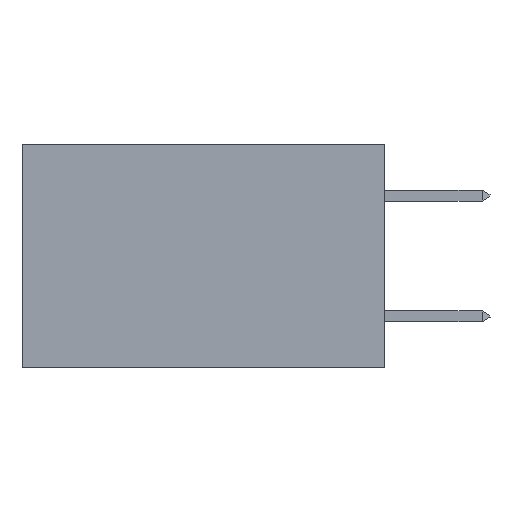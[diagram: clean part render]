
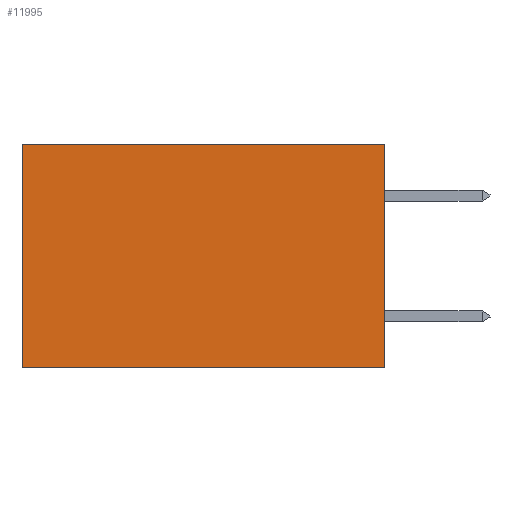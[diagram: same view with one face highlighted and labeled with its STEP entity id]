
A CAD part, left-side view. The second image highlights one B-rep face of the part: STEP entity #11995.
In plain terms, the highlighted planar face has unit normal (-1, 0, 0).
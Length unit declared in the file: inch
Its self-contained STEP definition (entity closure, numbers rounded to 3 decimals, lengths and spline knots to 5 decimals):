
#95 = AXIS2_PLACEMENT_3D ( 'NONE', #9193, #17863, #21063 ) ;
#186 = VERTEX_POINT ( 'NONE', #576 ) ;
#576 = CARTESIAN_POINT ( 'NONE',  ( 0.2875, 0.6, 0. ) ) ;
#880 = ORIENTED_EDGE ( 'NONE', *, *, #10664, .T. ) ;
#1171 = CARTESIAN_POINT ( 'NONE',  ( 0.2875, 0., -0.37 ) ) ;
#1989 = DIRECTION ( 'NONE',  ( 0., 1., 0. ) ) ;
#2350 = LINE ( 'NONE', #20956, #8080 ) ;
#3110 = DIRECTION ( 'NONE',  ( 0., 1., 0. ) ) ;
#3612 = LINE ( 'NONE', #1171, #22007 ) ;
#3798 = ORIENTED_EDGE ( 'NONE', *, *, #13768, .F. ) ;
#3937 = FACE_OUTER_BOUND ( 'NONE', #5094, .T. ) ;
#4368 = VERTEX_POINT ( 'NONE', #5726 ) ;
#5094 = EDGE_LOOP ( 'NONE', ( #7578, #20867, #3798, #880 ) ) ;
#5726 = CARTESIAN_POINT ( 'NONE',  ( 0.2875, 0., -0.37 ) ) ;
#6309 = CARTESIAN_POINT ( 'NONE',  ( 0.2875, 0.6, 0. ) ) ;
#7578 = ORIENTED_EDGE ( 'NONE', *, *, #9660, .T. ) ;
#8080 = VECTOR ( 'NONE', #1989, 39.37008 ) ;
#9193 = CARTESIAN_POINT ( 'NONE',  ( 0.2875, 0., 0. ) ) ;
#9660 = EDGE_CURVE ( 'NONE', #186, #22187, #11648, .T. ) ;
#9897 = DIRECTION ( 'NONE',  ( 0., 0., -1. ) ) ;
#10286 = CARTESIAN_POINT ( 'NONE',  ( 0.2875, 0.6, -0.37 ) ) ;
#10535 = CARTESIAN_POINT ( 'NONE',  ( 0.2875, 0., 0. ) ) ;
#10664 = EDGE_CURVE ( 'NONE', #13158, #186, #2350, .T. ) ;
#11648 = LINE ( 'NONE', #6309, #12415 ) ;
#11995 = ADVANCED_FACE ( 'NONE', ( #3937 ), #12548, .F. ) ;
#12415 = VECTOR ( 'NONE', #9897, 39.37008 ) ;
#12548 = PLANE ( 'NONE',  #95 ) ;
#13009 = EDGE_CURVE ( 'NONE', #4368, #22187, #3612, .T. ) ;
#13158 = VERTEX_POINT ( 'NONE', #17076 ) ;
#13768 = EDGE_CURVE ( 'NONE', #13158, #4368, #19886, .T. ) ;
#15314 = VECTOR ( 'NONE', #15559, 39.37008 ) ;
#15559 = DIRECTION ( 'NONE',  ( 0., 0., -1. ) ) ;
#17076 = CARTESIAN_POINT ( 'NONE',  ( 0.2875, 0., 0. ) ) ;
#17863 = DIRECTION ( 'NONE',  ( 1., 0., 0. ) ) ;
#19886 = LINE ( 'NONE', #10535, #15314 ) ;
#20867 = ORIENTED_EDGE ( 'NONE', *, *, #13009, .F. ) ;
#20956 = CARTESIAN_POINT ( 'NONE',  ( 0.2875, 0., 0. ) ) ;
#21063 = DIRECTION ( 'NONE',  ( 0., 0., -1. ) ) ;
#22007 = VECTOR ( 'NONE', #3110, 39.37008 ) ;
#22187 = VERTEX_POINT ( 'NONE', #10286 ) ;
